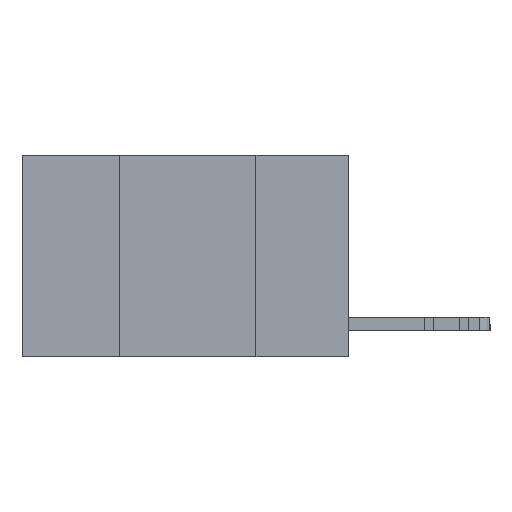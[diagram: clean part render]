
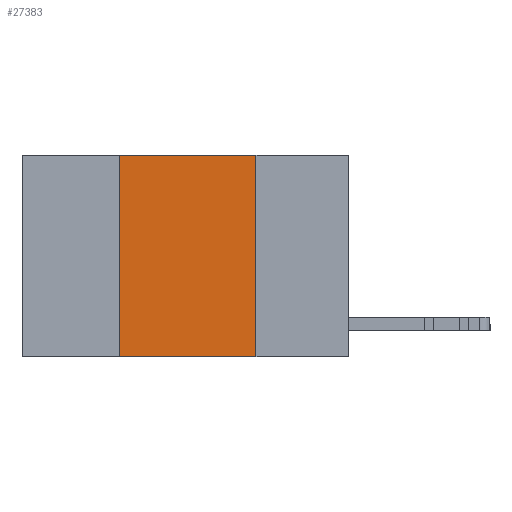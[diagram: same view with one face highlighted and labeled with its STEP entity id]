
A CAD part, left-side view. The second image highlights one B-rep face of the part: STEP entity #27383.
In plain terms, the highlighted planar face has unit normal (-1, 0, 0).
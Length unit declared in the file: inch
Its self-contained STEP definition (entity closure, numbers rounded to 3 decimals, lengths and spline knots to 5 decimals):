
#660 = CARTESIAN_POINT ( 'NONE',  ( 0., 0.6, 0. ) ) ;
#2420 = CARTESIAN_POINT ( 'NONE',  ( 0., 0.6, 0. ) ) ;
#2512 = EDGE_LOOP ( 'NONE', ( #28048, #7778, #29117, #8494 ) ) ;
#6080 = VERTEX_POINT ( 'NONE', #10377 ) ;
#6994 = CARTESIAN_POINT ( 'NONE',  ( 0., 0.42, -0.37 ) ) ;
#7324 = EDGE_CURVE ( 'NONE', #15259, #20640, #14139, .T. ) ;
#7778 = ORIENTED_EDGE ( 'NONE', *, *, #13322, .F. ) ;
#7913 = DIRECTION ( 'NONE',  ( 0., 0., -1. ) ) ;
#8494 = ORIENTED_EDGE ( 'NONE', *, *, #17466, .T. ) ;
#9185 = DIRECTION ( 'NONE',  ( 0., -1., 0. ) ) ;
#9210 = FACE_OUTER_BOUND ( 'NONE', #2512, .T. ) ;
#9357 = DIRECTION ( 'NONE',  ( 0., 0., -1. ) ) ;
#9491 = DIRECTION ( 'NONE',  ( 0., 0., 1. ) ) ;
#9789 = CARTESIAN_POINT ( 'NONE',  ( 0., 0.42, 0. ) ) ;
#9858 = DIRECTION ( 'NONE',  ( 0., -1., 0. ) ) ;
#10377 = CARTESIAN_POINT ( 'NONE',  ( 0., 0.17, 0. ) ) ;
#13322 = EDGE_CURVE ( 'NONE', #20640, #6080, #16616, .T. ) ;
#13991 = VECTOR ( 'NONE', #9491, 39.37008 ) ;
#14139 = LINE ( 'NONE', #9789, #13991 ) ;
#15204 = VECTOR ( 'NONE', #7913, 39.37008 ) ;
#15205 = CARTESIAN_POINT ( 'NONE',  ( 0., 0.17, -0.37 ) ) ;
#15259 = VERTEX_POINT ( 'NONE', #6994 ) ;
#16341 = VECTOR ( 'NONE', #9185, 39.37008 ) ;
#16616 = LINE ( 'NONE', #660, #24410 ) ;
#17466 = EDGE_CURVE ( 'NONE', #15259, #24519, #18793, .T. ) ;
#18793 = LINE ( 'NONE', #27830, #16341 ) ;
#19147 = AXIS2_PLACEMENT_3D ( 'NONE', #2420, #20787, #9357 ) ;
#20640 = VERTEX_POINT ( 'NONE', #25302 ) ;
#20787 = DIRECTION ( 'NONE',  ( 1., 0., 0. ) ) ;
#23995 = LINE ( 'NONE', #28515, #15204 ) ;
#24410 = VECTOR ( 'NONE', #9858, 39.37008 ) ;
#24519 = VERTEX_POINT ( 'NONE', #15205 ) ;
#25249 = EDGE_CURVE ( 'NONE', #6080, #24519, #23995, .T. ) ;
#25285 = PLANE ( 'NONE',  #19147 ) ;
#25302 = CARTESIAN_POINT ( 'NONE',  ( 0., 0.42, 0. ) ) ;
#27383 = ADVANCED_FACE ( 'NONE', ( #9210 ), #25285, .F. ) ;
#27830 = CARTESIAN_POINT ( 'NONE',  ( 0., 0.6, -0.37 ) ) ;
#28048 = ORIENTED_EDGE ( 'NONE', *, *, #25249, .F. ) ;
#28515 = CARTESIAN_POINT ( 'NONE',  ( 0., 0.17, 0. ) ) ;
#29117 = ORIENTED_EDGE ( 'NONE', *, *, #7324, .F. ) ;
